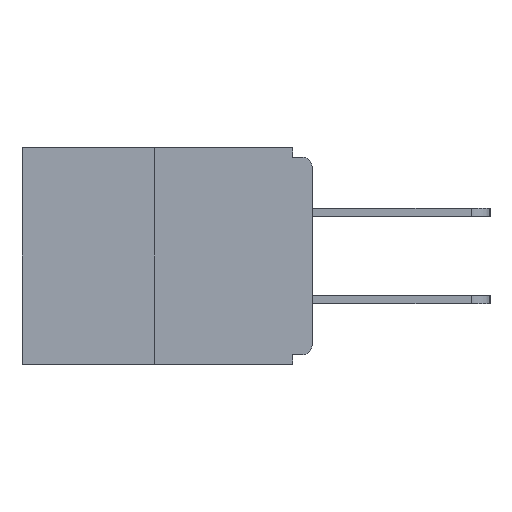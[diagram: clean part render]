
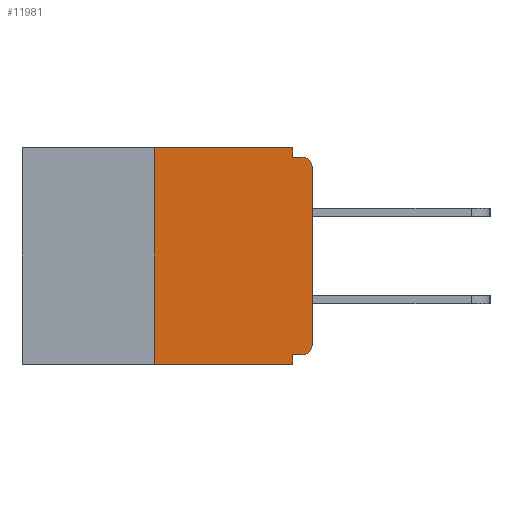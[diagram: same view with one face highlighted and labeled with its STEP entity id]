
A CAD part, left-side view. The second image highlights one B-rep face of the part: STEP entity #11981.
In plain terms, the highlighted planar face has unit normal (-1, 0, 0).
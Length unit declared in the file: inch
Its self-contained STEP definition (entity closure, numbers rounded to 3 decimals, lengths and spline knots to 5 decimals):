
#130 = DIRECTION ( 'NONE',  ( 0., 0., -1. ) ) ;
#325 = CIRCLE ( 'NONE', #2312, 0.015 ) ;
#1097 = LINE ( 'NONE', #22137, #17308 ) ;
#1107 = VERTEX_POINT ( 'NONE', #11228 ) ;
#1168 = VECTOR ( 'NONE', #130, 39.37008 ) ;
#1896 = DIRECTION ( 'NONE',  ( 0., 0., -1. ) ) ;
#2014 = CARTESIAN_POINT ( 'NONE',  ( 0., 0.031, 0. ) ) ;
#2195 = LINE ( 'NONE', #17001, #4006 ) ;
#2312 = AXIS2_PLACEMENT_3D ( 'NONE', #13180, #3517, #24470 ) ;
#2382 = VECTOR ( 'NONE', #7705, 39.37008 ) ;
#2701 = LINE ( 'NONE', #8464, #21120 ) ;
#2986 = LINE ( 'NONE', #8747, #13109 ) ;
#3517 = DIRECTION ( 'NONE',  ( -1., 0., 0. ) ) ;
#4006 = VECTOR ( 'NONE', #24645, 39.37008 ) ;
#4599 = CARTESIAN_POINT ( 'NONE',  ( 0., 0.015, -0.313 ) ) ;
#4696 = ORIENTED_EDGE ( 'NONE', *, *, #16174, .F. ) ;
#4881 = ORIENTED_EDGE ( 'NONE', *, *, #23011, .T. ) ;
#5139 = CARTESIAN_POINT ( 'NONE',  ( 0., 0., -0.313 ) ) ;
#5442 = VERTEX_POINT ( 'NONE', #8978 ) ;
#5483 = EDGE_CURVE ( 'NONE', #17661, #20365, #1097, .T. ) ;
#5701 = VERTEX_POINT ( 'NONE', #18324 ) ;
#6009 = CARTESIAN_POINT ( 'NONE',  ( 0., 0.46, 0. ) ) ;
#6443 = ORIENTED_EDGE ( 'NONE', *, *, #19387, .T. ) ;
#6629 = EDGE_CURVE ( 'NONE', #5701, #8958, #14342, .T. ) ;
#7075 = ORIENTED_EDGE ( 'NONE', *, *, #6629, .T. ) ;
#7393 = DIRECTION ( 'NONE',  ( 1., 0., 0. ) ) ;
#7551 = DIRECTION ( 'NONE',  ( 0., 0., 1. ) ) ;
#7705 = DIRECTION ( 'NONE',  ( 0., -1., 0. ) ) ;
#7723 = CARTESIAN_POINT ( 'NONE',  ( 0., 0.031, -0.343 ) ) ;
#8113 = DIRECTION ( 'NONE',  ( -1., 0., 0. ) ) ;
#8241 = ORIENTED_EDGE ( 'NONE', *, *, #24458, .F. ) ;
#8341 = AXIS2_PLACEMENT_3D ( 'NONE', #4599, #8113, #23557 ) ;
#8464 = CARTESIAN_POINT ( 'NONE',  ( 0., 0., -0.328 ) ) ;
#8718 = DIRECTION ( 'NONE',  ( 0., -1., 0. ) ) ;
#8747 = CARTESIAN_POINT ( 'NONE',  ( 0., 0., -0.015 ) ) ;
#8958 = VERTEX_POINT ( 'NONE', #5139 ) ;
#8978 = CARTESIAN_POINT ( 'NONE',  ( 0., 0.031, -0.343 ) ) ;
#9326 = CARTESIAN_POINT ( 'NONE',  ( 0., 0.015, -0.015 ) ) ;
#11049 = FACE_OUTER_BOUND ( 'NONE', #18649, .T. ) ;
#11228 = CARTESIAN_POINT ( 'NONE',  ( 0., 0.031, -0.328 ) ) ;
#11395 = VERTEX_POINT ( 'NONE', #9326 ) ;
#11554 = ORIENTED_EDGE ( 'NONE', *, *, #16592, .F. ) ;
#11981 = ADVANCED_FACE ( 'NONE', ( #11049 ), #18701, .F. ) ;
#12095 = AXIS2_PLACEMENT_3D ( 'NONE', #6009, #7393, #1896 ) ;
#12903 = EDGE_CURVE ( 'NONE', #16839, #17661, #17474, .T. ) ;
#13109 = VECTOR ( 'NONE', #16402, 39.37008 ) ;
#13180 = CARTESIAN_POINT ( 'NONE',  ( 0., 0.015, -0.03 ) ) ;
#13608 = CARTESIAN_POINT ( 'NONE',  ( 0., 0.031, 0. ) ) ;
#14342 = CIRCLE ( 'NONE', #8341, 0.015 ) ;
#14531 = VERTEX_POINT ( 'NONE', #16019 ) ;
#15144 = ORIENTED_EDGE ( 'NONE', *, *, #18130, .F. ) ;
#15162 = ORIENTED_EDGE ( 'NONE', *, *, #5483, .F. ) ;
#15305 = LINE ( 'NONE', #2014, #1168 ) ;
#16019 = CARTESIAN_POINT ( 'NONE',  ( 0., 0.031, -0.015 ) ) ;
#16174 = EDGE_CURVE ( 'NONE', #14531, #11395, #2986, .T. ) ;
#16402 = DIRECTION ( 'NONE',  ( 0., -1., 0. ) ) ;
#16592 = EDGE_CURVE ( 'NONE', #5701, #1107, #2701, .T. ) ;
#16839 = VERTEX_POINT ( 'NONE', #22900 ) ;
#16924 = LINE ( 'NONE', #18930, #2382 ) ;
#16972 = ORIENTED_EDGE ( 'NONE', *, *, #12903, .F. ) ;
#17001 = CARTESIAN_POINT ( 'NONE',  ( 0., 0., 0. ) ) ;
#17308 = VECTOR ( 'NONE', #8718, 39.37008 ) ;
#17474 = LINE ( 'NONE', #20971, #23413 ) ;
#17661 = VERTEX_POINT ( 'NONE', #19706 ) ;
#18100 = DIRECTION ( 'NONE',  ( 0., 0., -1. ) ) ;
#18130 = EDGE_CURVE ( 'NONE', #20365, #14531, #15305, .T. ) ;
#18324 = CARTESIAN_POINT ( 'NONE',  ( 0., 0.015, -0.328 ) ) ;
#18524 = DIRECTION ( 'NONE',  ( 0., 1., 0. ) ) ;
#18649 = EDGE_LOOP ( 'NONE', ( #15162, #16972, #20801, #8241, #11554, #7075, #4881, #6443, #4696, #15144 ) ) ;
#18701 = PLANE ( 'NONE',  #12095 ) ;
#18890 = VECTOR ( 'NONE', #18100, 39.37008 ) ;
#18930 = CARTESIAN_POINT ( 'NONE',  ( 0., 0.46, -0.343 ) ) ;
#19018 = CARTESIAN_POINT ( 'NONE',  ( 0., 0., -0.03 ) ) ;
#19387 = EDGE_CURVE ( 'NONE', #20340, #11395, #325, .T. ) ;
#19706 = CARTESIAN_POINT ( 'NONE',  ( 0., 0.25, 0. ) ) ;
#20340 = VERTEX_POINT ( 'NONE', #19018 ) ;
#20365 = VERTEX_POINT ( 'NONE', #13608 ) ;
#20801 = ORIENTED_EDGE ( 'NONE', *, *, #21093, .T. ) ;
#20971 = CARTESIAN_POINT ( 'NONE',  ( 0., 0.25, 0. ) ) ;
#21093 = EDGE_CURVE ( 'NONE', #16839, #5442, #16924, .T. ) ;
#21120 = VECTOR ( 'NONE', #18524, 39.37008 ) ;
#21397 = LINE ( 'NONE', #7723, #18890 ) ;
#22137 = CARTESIAN_POINT ( 'NONE',  ( 0., 0.46, 0. ) ) ;
#22900 = CARTESIAN_POINT ( 'NONE',  ( 0., 0.25, -0.343 ) ) ;
#23011 = EDGE_CURVE ( 'NONE', #8958, #20340, #2195, .T. ) ;
#23413 = VECTOR ( 'NONE', #7551, 39.37008 ) ;
#23557 = DIRECTION ( 'NONE',  ( 0., 0., -1. ) ) ;
#24458 = EDGE_CURVE ( 'NONE', #1107, #5442, #21397, .T. ) ;
#24470 = DIRECTION ( 'NONE',  ( 0., 0., -1. ) ) ;
#24645 = DIRECTION ( 'NONE',  ( 0., 0., 1. ) ) ;
